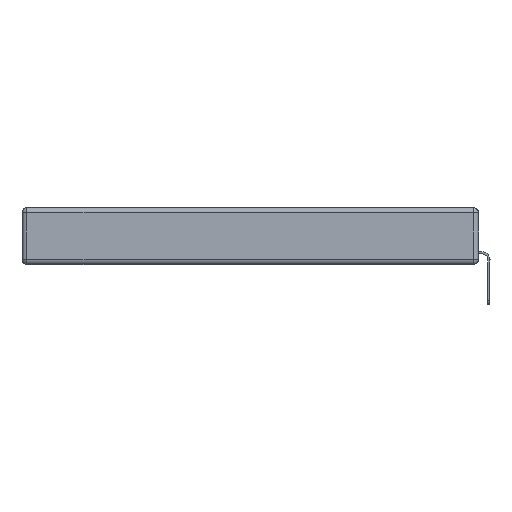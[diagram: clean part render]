
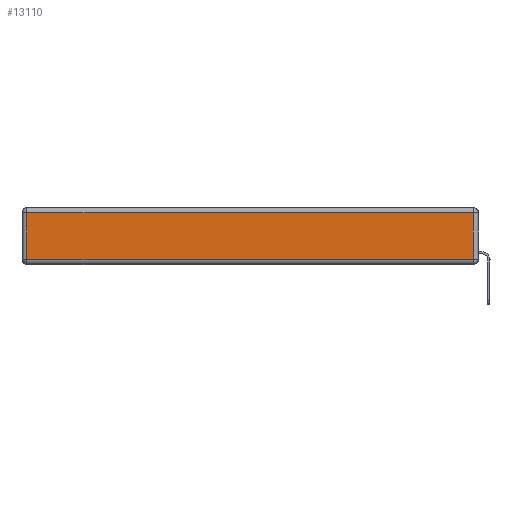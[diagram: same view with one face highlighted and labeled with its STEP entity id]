
A CAD part, left-side view. The second image highlights one B-rep face of the part: STEP entity #13110.
In plain terms, the highlighted planar face has unit normal (-1, 0, 0).
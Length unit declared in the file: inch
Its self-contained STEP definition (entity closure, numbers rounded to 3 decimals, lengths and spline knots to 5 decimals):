
#977 = DIRECTION ( 'NONE',  ( 0., 0., 1. ) ) ;
#1778 = CARTESIAN_POINT ( 'NONE',  ( 0., 0.03, -0.343 ) ) ;
#2453 = DIRECTION ( 'NONE',  ( -1., 0., 0. ) ) ;
#3497 = VERTEX_POINT ( 'NONE', #11641 ) ;
#3987 = LINE ( 'NONE', #9676, #11520 ) ;
#4206 = EDGE_CURVE ( 'NONE', #6553, #3497, #3987, .T. ) ;
#5101 = DIRECTION ( 'NONE',  ( 0., 0., -1. ) ) ;
#5582 = VECTOR ( 'NONE', #15692, 39.37008 ) ;
#5664 = DIRECTION ( 'NONE',  ( 0., 1., 0. ) ) ;
#5744 = EDGE_CURVE ( 'NONE', #3497, #15117, #14829, .T. ) ;
#6507 = CARTESIAN_POINT ( 'NONE',  ( 0., 2.72, -0.343 ) ) ;
#6553 = VERTEX_POINT ( 'NONE', #13590 ) ;
#7356 = LINE ( 'NONE', #1778, #5582 ) ;
#7493 = CARTESIAN_POINT ( 'NONE',  ( 0., 0., -0.313 ) ) ;
#7587 = CARTESIAN_POINT ( 'NONE',  ( 0., 0.03, -0.313 ) ) ;
#8217 = PLANE ( 'NONE',  #12980 ) ;
#8567 = CARTESIAN_POINT ( 'NONE',  ( 0., 2.72, -0.313 ) ) ;
#9230 = ORIENTED_EDGE ( 'NONE', *, *, #15023, .T. ) ;
#9676 = CARTESIAN_POINT ( 'NONE',  ( 0., 2.75, -0.03 ) ) ;
#9717 = FACE_OUTER_BOUND ( 'NONE', #15100, .T. ) ;
#10001 = VECTOR ( 'NONE', #15643, 39.37008 ) ;
#10012 = LINE ( 'NONE', #7493, #10001 ) ;
#10529 = ORIENTED_EDGE ( 'NONE', *, *, #11577, .T. ) ;
#11520 = VECTOR ( 'NONE', #5664, 39.37008 ) ;
#11577 = EDGE_CURVE ( 'NONE', #15117, #14693, #10012, .T. ) ;
#11641 = CARTESIAN_POINT ( 'NONE',  ( 0., 2.72, -0.03 ) ) ;
#12980 = AXIS2_PLACEMENT_3D ( 'NONE', #13692, #2453, #977 ) ;
#13110 = ADVANCED_FACE ( 'NONE', ( #9717 ), #8217, .T. ) ;
#13590 = CARTESIAN_POINT ( 'NONE',  ( 0., 0.03, -0.03 ) ) ;
#13692 = CARTESIAN_POINT ( 'NONE',  ( 0., 0., -0.343 ) ) ;
#14693 = VERTEX_POINT ( 'NONE', #7587 ) ;
#14829 = LINE ( 'NONE', #6507, #15905 ) ;
#15023 = EDGE_CURVE ( 'NONE', #14693, #6553, #7356, .T. ) ;
#15100 = EDGE_LOOP ( 'NONE', ( #10529, #9230, #17348, #16320 ) ) ;
#15117 = VERTEX_POINT ( 'NONE', #8567 ) ;
#15643 = DIRECTION ( 'NONE',  ( 0., -1., 0. ) ) ;
#15692 = DIRECTION ( 'NONE',  ( 0., 0., 1. ) ) ;
#15905 = VECTOR ( 'NONE', #5101, 39.37008 ) ;
#16320 = ORIENTED_EDGE ( 'NONE', *, *, #5744, .T. ) ;
#17348 = ORIENTED_EDGE ( 'NONE', *, *, #4206, .T. ) ;
